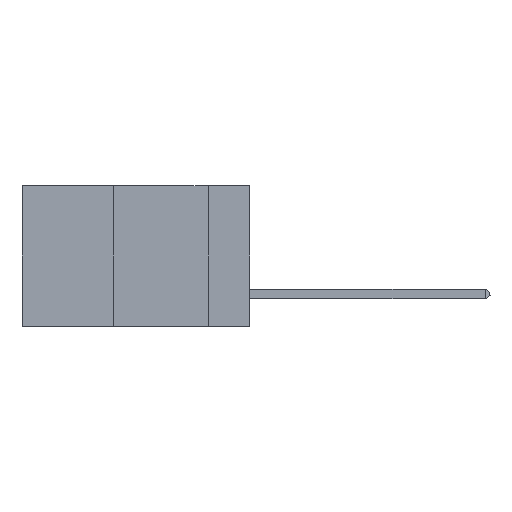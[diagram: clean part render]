
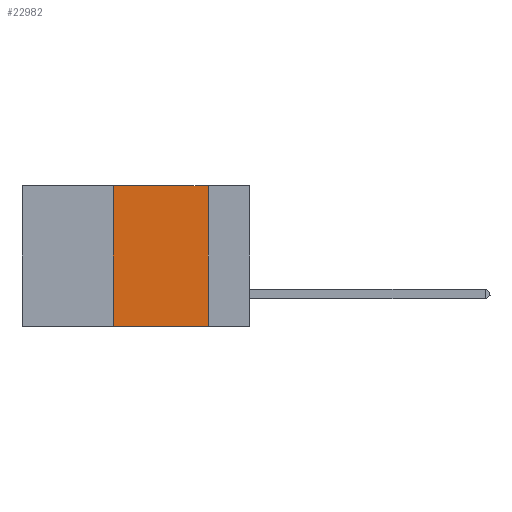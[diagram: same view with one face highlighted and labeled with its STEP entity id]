
A CAD part, left-side view. The second image highlights one B-rep face of the part: STEP entity #22982.
In plain terms, the highlighted planar face has unit normal (-1, 0, 0).
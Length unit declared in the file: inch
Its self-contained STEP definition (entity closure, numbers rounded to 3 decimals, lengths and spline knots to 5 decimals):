
#2709 = VECTOR ( 'NONE', #23899, 39.37008 ) ;
#4419 = CARTESIAN_POINT ( 'NONE',  ( 0., 0.11, 0. ) ) ;
#5014 = LINE ( 'NONE', #8227, #20044 ) ;
#5284 = DIRECTION ( 'NONE',  ( 0., -1., 0. ) ) ;
#5331 = VERTEX_POINT ( 'NONE', #16522 ) ;
#5370 = CARTESIAN_POINT ( 'NONE',  ( 0., 0.11, -0.37 ) ) ;
#8007 = CARTESIAN_POINT ( 'NONE',  ( 0., 0.6, -0.37 ) ) ;
#8227 = CARTESIAN_POINT ( 'NONE',  ( 0., 0.36, 0. ) ) ;
#11324 = EDGE_CURVE ( 'NONE', #18283, #17844, #5014, .T. ) ;
#11633 = EDGE_CURVE ( 'NONE', #18283, #28583, #29354, .T. ) ;
#12370 = EDGE_CURVE ( 'NONE', #5331, #28583, #31499, .T. ) ;
#13663 = ORIENTED_EDGE ( 'NONE', *, *, #17189, .F. ) ;
#13804 = ORIENTED_EDGE ( 'NONE', *, *, #11633, .T. ) ;
#15645 = CARTESIAN_POINT ( 'NONE',  ( 0., 0.6, 0. ) ) ;
#16522 = CARTESIAN_POINT ( 'NONE',  ( 0., 0.11, 0. ) ) ;
#17189 = EDGE_CURVE ( 'NONE', #17844, #5331, #24525, .T. ) ;
#17388 = DIRECTION ( 'NONE',  ( 0., 0., 1. ) ) ;
#17844 = VERTEX_POINT ( 'NONE', #33130 ) ;
#18216 = DIRECTION ( 'NONE',  ( 1., 0., 0. ) ) ;
#18283 = VERTEX_POINT ( 'NONE', #35300 ) ;
#20044 = VECTOR ( 'NONE', #17388, 39.37008 ) ;
#20672 = DIRECTION ( 'NONE',  ( 0., 0., -1. ) ) ;
#22982 = ADVANCED_FACE ( 'NONE', ( #26132 ), #29509, .F. ) ;
#23899 = DIRECTION ( 'NONE',  ( 0., 0., -1. ) ) ;
#24525 = LINE ( 'NONE', #33517, #32899 ) ;
#24558 = DIRECTION ( 'NONE',  ( 0., -1., 0. ) ) ;
#26132 = FACE_OUTER_BOUND ( 'NONE', #27976, .T. ) ;
#27976 = EDGE_LOOP ( 'NONE', ( #34221, #13663, #35442, #13804 ) ) ;
#28452 = VECTOR ( 'NONE', #24558, 39.37008 ) ;
#28583 = VERTEX_POINT ( 'NONE', #5370 ) ;
#29354 = LINE ( 'NONE', #8007, #28452 ) ;
#29509 = PLANE ( 'NONE',  #36341 ) ;
#31499 = LINE ( 'NONE', #4419, #2709 ) ;
#32899 = VECTOR ( 'NONE', #5284, 39.37008 ) ;
#33130 = CARTESIAN_POINT ( 'NONE',  ( 0., 0.36, 0. ) ) ;
#33517 = CARTESIAN_POINT ( 'NONE',  ( 0., 0.6, 0. ) ) ;
#34221 = ORIENTED_EDGE ( 'NONE', *, *, #12370, .F. ) ;
#35300 = CARTESIAN_POINT ( 'NONE',  ( 0., 0.36, -0.37 ) ) ;
#35442 = ORIENTED_EDGE ( 'NONE', *, *, #11324, .F. ) ;
#36341 = AXIS2_PLACEMENT_3D ( 'NONE', #15645, #18216, #20672 ) ;
